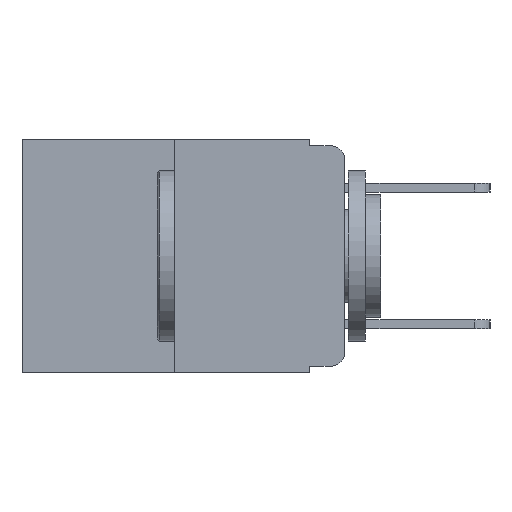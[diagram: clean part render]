
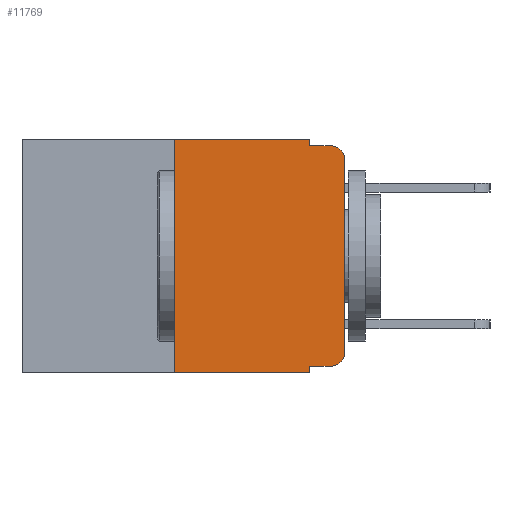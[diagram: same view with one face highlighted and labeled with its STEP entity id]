
A CAD part, left-side view. The second image highlights one B-rep face of the part: STEP entity #11769.
In plain terms, the highlighted planar face has unit normal (-1, 0, 0).
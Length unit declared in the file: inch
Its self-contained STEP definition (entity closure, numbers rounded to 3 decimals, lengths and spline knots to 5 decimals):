
#30 = EDGE_CURVE ( 'NONE', #13282, #8813, #11981, .T. ) ;
#155 = ORIENTED_EDGE ( 'NONE', *, *, #6232, .F. ) ;
#378 = VECTOR ( 'NONE', #9266, 39.37008 ) ;
#654 = DIRECTION ( 'NONE',  ( 0., 0., -1. ) ) ;
#660 = CARTESIAN_POINT ( 'NONE',  ( 0., 0.25, -0.343 ) ) ;
#756 = DIRECTION ( 'NONE',  ( -1., 0., 0. ) ) ;
#925 = DIRECTION ( 'NONE',  ( 0., -1., 0. ) ) ;
#976 = VECTOR ( 'NONE', #4764, 39.37008 ) ;
#1490 = EDGE_CURVE ( 'NONE', #7528, #9341, #5556, .T. ) ;
#1712 = VECTOR ( 'NONE', #654, 39.37008 ) ;
#1771 = EDGE_CURVE ( 'NONE', #3078, #18655, #8274, .T. ) ;
#1962 = CARTESIAN_POINT ( 'NONE',  ( 0., 0.473, 0. ) ) ;
#2019 = CARTESIAN_POINT ( 'NONE',  ( 0., 0.25, 0. ) ) ;
#2743 = AXIS2_PLACEMENT_3D ( 'NONE', #9454, #756, #10926 ) ;
#3078 = VERTEX_POINT ( 'NONE', #6315 ) ;
#3234 = EDGE_CURVE ( 'NONE', #3078, #6481, #9865, .T. ) ;
#3260 = CARTESIAN_POINT ( 'NONE',  ( 0., 0.02, -0.333 ) ) ;
#3325 = CARTESIAN_POINT ( 'NONE',  ( 0., 0.051, -0.01 ) ) ;
#3474 = DIRECTION ( 'NONE',  ( 1., 0., 0. ) ) ;
#3528 = ORIENTED_EDGE ( 'NONE', *, *, #3234, .T. ) ;
#4460 = VERTEX_POINT ( 'NONE', #14284 ) ;
#4545 = CARTESIAN_POINT ( 'NONE',  ( 0., 0.473, -0.343 ) ) ;
#4702 = DIRECTION ( 'NONE',  ( -1., 0., 0. ) ) ;
#4764 = DIRECTION ( 'NONE',  ( 0., -1., 0. ) ) ;
#5224 = CARTESIAN_POINT ( 'NONE',  ( 0., 0.051, -0.333 ) ) ;
#5232 = ORIENTED_EDGE ( 'NONE', *, *, #12664, .T. ) ;
#5278 = CIRCLE ( 'NONE', #7702, 0.02 ) ;
#5556 = LINE ( 'NONE', #6432, #1712 ) ;
#5720 = DIRECTION ( 'NONE',  ( 0., 0., -1. ) ) ;
#5953 = VECTOR ( 'NONE', #10220, 39.37008 ) ;
#5984 = VECTOR ( 'NONE', #925, 39.37008 ) ;
#5996 = CARTESIAN_POINT ( 'NONE',  ( 0., 0.051, -0.01 ) ) ;
#6232 = EDGE_CURVE ( 'NONE', #8813, #7528, #14439, .T. ) ;
#6315 = CARTESIAN_POINT ( 'NONE',  ( 0., 0.051, -0.333 ) ) ;
#6432 = CARTESIAN_POINT ( 'NONE',  ( 0., 0.051, 0. ) ) ;
#6481 = VERTEX_POINT ( 'NONE', #3260 ) ;
#6645 = LINE ( 'NONE', #4545, #17794 ) ;
#6772 = FACE_OUTER_BOUND ( 'NONE', #10881, .T. ) ;
#7263 = VERTEX_POINT ( 'NONE', #16623 ) ;
#7528 = VERTEX_POINT ( 'NONE', #14316 ) ;
#7702 = AXIS2_PLACEMENT_3D ( 'NONE', #13432, #4702, #14895 ) ;
#7738 = AXIS2_PLACEMENT_3D ( 'NONE', #1962, #3474, #13631 ) ;
#7911 = EDGE_CURVE ( 'NONE', #4460, #7263, #18018, .T. ) ;
#8193 = ORIENTED_EDGE ( 'NONE', *, *, #12416, .T. ) ;
#8274 = LINE ( 'NONE', #14433, #12159 ) ;
#8314 = VERTEX_POINT ( 'NONE', #16927 ) ;
#8800 = ORIENTED_EDGE ( 'NONE', *, *, #1490, .F. ) ;
#8813 = VERTEX_POINT ( 'NONE', #10772 ) ;
#9266 = DIRECTION ( 'NONE',  ( 0., 0., 1. ) ) ;
#9341 = VERTEX_POINT ( 'NONE', #5996 ) ;
#9404 = EDGE_CURVE ( 'NONE', #7263, #8314, #5278, .T. ) ;
#9436 = EDGE_CURVE ( 'NONE', #9341, #8314, #12130, .T. ) ;
#9454 = CARTESIAN_POINT ( 'NONE',  ( 0., 0.02, -0.313 ) ) ;
#9865 = LINE ( 'NONE', #5224, #5984 ) ;
#10184 = CARTESIAN_POINT ( 'NONE',  ( 0., 0.051, -0.343 ) ) ;
#10220 = DIRECTION ( 'NONE',  ( 0., 0., 1. ) ) ;
#10299 = CIRCLE ( 'NONE', #2743, 0.02 ) ;
#10601 = VECTOR ( 'NONE', #15602, 39.37008 ) ;
#10772 = CARTESIAN_POINT ( 'NONE',  ( 0., 0.25, 0. ) ) ;
#10881 = EDGE_LOOP ( 'NONE', ( #14893, #18069, #13174, #8800, #155, #18265, #8193, #12276, #3528, #5232 ) ) ;
#10926 = DIRECTION ( 'NONE',  ( 0., 0., -1. ) ) ;
#11694 = CARTESIAN_POINT ( 'NONE',  ( 0., 0., 0. ) ) ;
#11769 = ADVANCED_FACE ( 'NONE', ( #6772 ), #12192, .F. ) ;
#11981 = LINE ( 'NONE', #2019, #378 ) ;
#12130 = LINE ( 'NONE', #3325, #976 ) ;
#12159 = VECTOR ( 'NONE', #5720, 39.37008 ) ;
#12192 = PLANE ( 'NONE',  #7738 ) ;
#12276 = ORIENTED_EDGE ( 'NONE', *, *, #1771, .F. ) ;
#12416 = EDGE_CURVE ( 'NONE', #13282, #18655, #6645, .T. ) ;
#12664 = EDGE_CURVE ( 'NONE', #6481, #4460, #10299, .T. ) ;
#13174 = ORIENTED_EDGE ( 'NONE', *, *, #9436, .F. ) ;
#13282 = VERTEX_POINT ( 'NONE', #660 ) ;
#13432 = CARTESIAN_POINT ( 'NONE',  ( 0., 0.02, -0.03 ) ) ;
#13631 = DIRECTION ( 'NONE',  ( 0., 0., -1. ) ) ;
#14284 = CARTESIAN_POINT ( 'NONE',  ( 0., 0., -0.313 ) ) ;
#14316 = CARTESIAN_POINT ( 'NONE',  ( 0., 0.051, 0. ) ) ;
#14433 = CARTESIAN_POINT ( 'NONE',  ( 0., 0.051, 0. ) ) ;
#14439 = LINE ( 'NONE', #17061, #10601 ) ;
#14721 = DIRECTION ( 'NONE',  ( 0., -1., 0. ) ) ;
#14893 = ORIENTED_EDGE ( 'NONE', *, *, #7911, .T. ) ;
#14895 = DIRECTION ( 'NONE',  ( 0., 0., -1. ) ) ;
#15602 = DIRECTION ( 'NONE',  ( 0., -1., 0. ) ) ;
#16623 = CARTESIAN_POINT ( 'NONE',  ( 0., 0., -0.03 ) ) ;
#16927 = CARTESIAN_POINT ( 'NONE',  ( 0., 0.02, -0.01 ) ) ;
#17061 = CARTESIAN_POINT ( 'NONE',  ( 0., 0.473, 0. ) ) ;
#17794 = VECTOR ( 'NONE', #14721, 39.37008 ) ;
#18018 = LINE ( 'NONE', #11694, #5953 ) ;
#18069 = ORIENTED_EDGE ( 'NONE', *, *, #9404, .T. ) ;
#18265 = ORIENTED_EDGE ( 'NONE', *, *, #30, .F. ) ;
#18655 = VERTEX_POINT ( 'NONE', #10184 ) ;
